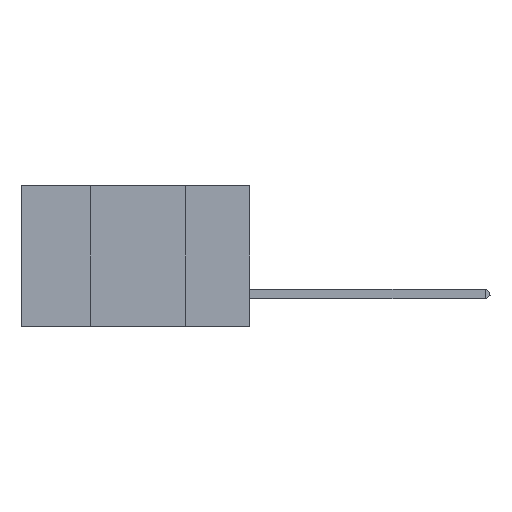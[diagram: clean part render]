
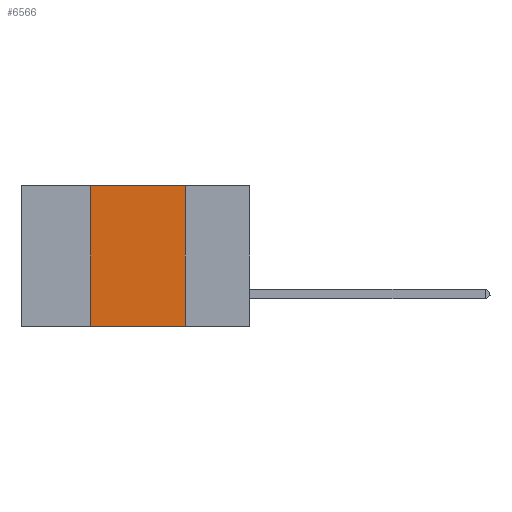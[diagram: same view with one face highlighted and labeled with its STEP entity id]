
A CAD part, left-side view. The second image highlights one B-rep face of the part: STEP entity #6566.
In plain terms, the highlighted planar face has unit normal (-1, 0, 0).
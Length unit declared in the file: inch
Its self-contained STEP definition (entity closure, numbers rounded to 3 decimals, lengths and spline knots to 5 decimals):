
#333 = CARTESIAN_POINT ( 'NONE',  ( 0., 0.6, 0. ) ) ;
#550 = EDGE_LOOP ( 'NONE', ( #1332, #13305, #17483, #4464 ) ) ;
#1186 = EDGE_CURVE ( 'NONE', #8726, #12328, #5230, .T. ) ;
#1332 = ORIENTED_EDGE ( 'NONE', *, *, #12258, .F. ) ;
#3070 = LINE ( 'NONE', #13001, #3963 ) ;
#3218 = VERTEX_POINT ( 'NONE', #8543 ) ;
#3272 = DIRECTION ( 'NONE',  ( 0., 0., -1. ) ) ;
#3776 = AXIS2_PLACEMENT_3D ( 'NONE', #333, #13296, #3272 ) ;
#3898 = LINE ( 'NONE', #4130, #18399 ) ;
#3963 = VECTOR ( 'NONE', #5839, 39.37008 ) ;
#4130 = CARTESIAN_POINT ( 'NONE',  ( 0., 0.17, 0. ) ) ;
#4464 = ORIENTED_EDGE ( 'NONE', *, *, #1186, .T. ) ;
#4524 = LINE ( 'NONE', #15647, #15361 ) ;
#5230 = LINE ( 'NONE', #15074, #10654 ) ;
#5839 = DIRECTION ( 'NONE',  ( 0., 0., 1. ) ) ;
#6566 = ADVANCED_FACE ( 'NONE', ( #14060 ), #13416, .F. ) ;
#7681 = DIRECTION ( 'NONE',  ( 0., -1., 0. ) ) ;
#8286 = VERTEX_POINT ( 'NONE', #11639 ) ;
#8543 = CARTESIAN_POINT ( 'NONE',  ( 0., 0.17, 0. ) ) ;
#8726 = VERTEX_POINT ( 'NONE', #16261 ) ;
#8861 = CARTESIAN_POINT ( 'NONE',  ( 0., 0.17, -0.37 ) ) ;
#10654 = VECTOR ( 'NONE', #7681, 39.37008 ) ;
#11639 = CARTESIAN_POINT ( 'NONE',  ( 0., 0.42, 0. ) ) ;
#12258 = EDGE_CURVE ( 'NONE', #3218, #12328, #3898, .T. ) ;
#12328 = VERTEX_POINT ( 'NONE', #8861 ) ;
#12830 = DIRECTION ( 'NONE',  ( 0., 0., -1. ) ) ;
#13001 = CARTESIAN_POINT ( 'NONE',  ( 0., 0.42, 0. ) ) ;
#13296 = DIRECTION ( 'NONE',  ( 1., 0., 0. ) ) ;
#13305 = ORIENTED_EDGE ( 'NONE', *, *, #17476, .F. ) ;
#13416 = PLANE ( 'NONE',  #3776 ) ;
#14060 = FACE_OUTER_BOUND ( 'NONE', #550, .T. ) ;
#14134 = EDGE_CURVE ( 'NONE', #8726, #8286, #3070, .T. ) ;
#15074 = CARTESIAN_POINT ( 'NONE',  ( 0., 0.6, -0.37 ) ) ;
#15361 = VECTOR ( 'NONE', #17134, 39.37008 ) ;
#15647 = CARTESIAN_POINT ( 'NONE',  ( 0., 0.6, 0. ) ) ;
#16261 = CARTESIAN_POINT ( 'NONE',  ( 0., 0.42, -0.37 ) ) ;
#17134 = DIRECTION ( 'NONE',  ( 0., -1., 0. ) ) ;
#17476 = EDGE_CURVE ( 'NONE', #8286, #3218, #4524, .T. ) ;
#17483 = ORIENTED_EDGE ( 'NONE', *, *, #14134, .F. ) ;
#18399 = VECTOR ( 'NONE', #12830, 39.37008 ) ;
